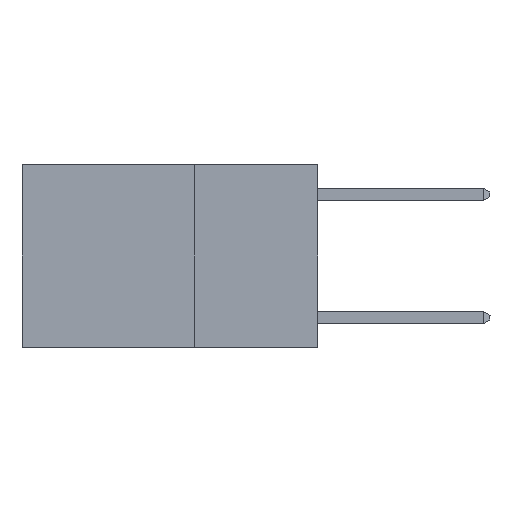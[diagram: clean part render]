
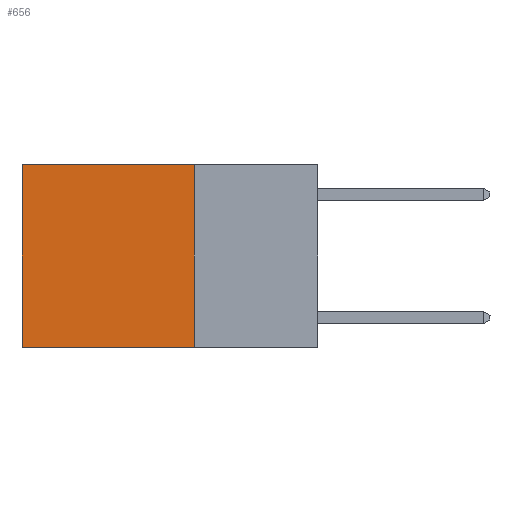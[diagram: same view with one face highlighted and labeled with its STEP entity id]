
A CAD part, left-side view. The second image highlights one B-rep face of the part: STEP entity #656.
In plain terms, the highlighted planar face has unit normal (-1, 0, 0).
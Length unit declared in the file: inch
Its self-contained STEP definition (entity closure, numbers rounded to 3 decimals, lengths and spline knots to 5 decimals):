
#58 = EDGE_CURVE ( 'NONE', #8360, #1944, #3573, .T. ) ;
#533 = EDGE_CURVE ( 'NONE', #1944, #9197, #3806, .T. ) ;
#656 = ADVANCED_FACE ( 'NONE', ( #2462 ), #1898, .F. ) ;
#970 = CARTESIAN_POINT ( 'NONE',  ( 0.2625, 0.25, 0. ) ) ;
#1059 = DIRECTION ( 'NONE',  ( 0., 0., -1. ) ) ;
#1098 = EDGE_CURVE ( 'NONE', #8360, #8141, #6563, .T. ) ;
#1845 = VECTOR ( 'NONE', #9657, 39.37008 ) ;
#1898 = PLANE ( 'NONE',  #8477 ) ;
#1944 = VERTEX_POINT ( 'NONE', #4827 ) ;
#2104 = DIRECTION ( 'NONE',  ( 0., 0., -1. ) ) ;
#2138 = CARTESIAN_POINT ( 'NONE',  ( 0.2625, 0.25, 0. ) ) ;
#2462 = FACE_OUTER_BOUND ( 'NONE', #7751, .T. ) ;
#3132 = VECTOR ( 'NONE', #6189, 39.37008 ) ;
#3400 = CARTESIAN_POINT ( 'NONE',  ( 0.2625, 0.6, 0. ) ) ;
#3436 = VECTOR ( 'NONE', #1059, 39.37008 ) ;
#3573 = LINE ( 'NONE', #7158, #3132 ) ;
#3806 = LINE ( 'NONE', #9463, #1845 ) ;
#4148 = CARTESIAN_POINT ( 'NONE',  ( 0.2625, 0.6, -0.37 ) ) ;
#4155 = DIRECTION ( 'NONE',  ( 1., 0., 0. ) ) ;
#4446 = CARTESIAN_POINT ( 'NONE',  ( 0.2625, 0.6, 0. ) ) ;
#4827 = CARTESIAN_POINT ( 'NONE',  ( 0.2625, 0.25, -0.37 ) ) ;
#6189 = DIRECTION ( 'NONE',  ( 0., 0., -1. ) ) ;
#6563 = LINE ( 'NONE', #9297, #6779 ) ;
#6615 = ORIENTED_EDGE ( 'NONE', *, *, #533, .F. ) ;
#6624 = ORIENTED_EDGE ( 'NONE', *, *, #58, .F. ) ;
#6779 = VECTOR ( 'NONE', #9415, 39.37008 ) ;
#6976 = ORIENTED_EDGE ( 'NONE', *, *, #8382, .T. ) ;
#7158 = CARTESIAN_POINT ( 'NONE',  ( 0.2625, 0.25, 0. ) ) ;
#7590 = ORIENTED_EDGE ( 'NONE', *, *, #1098, .T. ) ;
#7751 = EDGE_LOOP ( 'NONE', ( #6976, #6615, #6624, #7590 ) ) ;
#8141 = VERTEX_POINT ( 'NONE', #3400 ) ;
#8360 = VERTEX_POINT ( 'NONE', #970 ) ;
#8382 = EDGE_CURVE ( 'NONE', #8141, #9197, #10074, .T. ) ;
#8477 = AXIS2_PLACEMENT_3D ( 'NONE', #2138, #4155, #2104 ) ;
#9197 = VERTEX_POINT ( 'NONE', #4148 ) ;
#9297 = CARTESIAN_POINT ( 'NONE',  ( 0.2625, 0.25, 0. ) ) ;
#9415 = DIRECTION ( 'NONE',  ( 0., 1., 0. ) ) ;
#9463 = CARTESIAN_POINT ( 'NONE',  ( 0.2625, 0.25, -0.37 ) ) ;
#9657 = DIRECTION ( 'NONE',  ( 0., 1., 0. ) ) ;
#10074 = LINE ( 'NONE', #4446, #3436 ) ;
